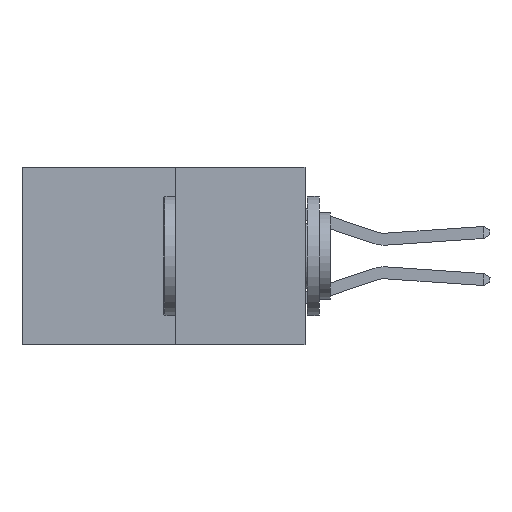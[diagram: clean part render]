
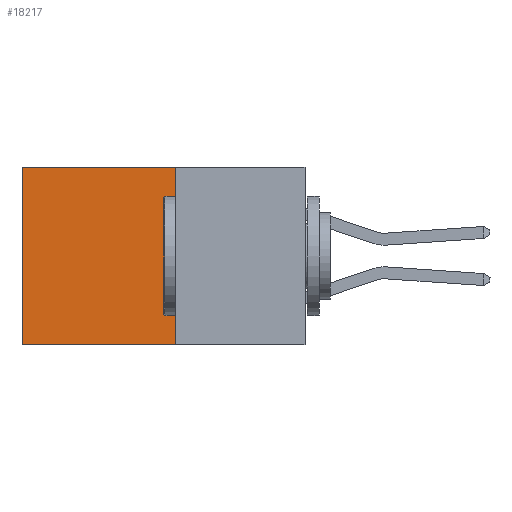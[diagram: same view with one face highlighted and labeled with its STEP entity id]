
A CAD part, left-side view. The second image highlights one B-rep face of the part: STEP entity #18217.
In plain terms, the highlighted planar face has unit normal (-1, 0, 0).
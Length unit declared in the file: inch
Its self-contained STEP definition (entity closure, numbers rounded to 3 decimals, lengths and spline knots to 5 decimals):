
#275 = LINE ( 'NONE', #4402, #13300 ) ;
#378 = VERTEX_POINT ( 'NONE', #5801 ) ;
#997 = EDGE_CURVE ( 'NONE', #378, #18207, #5376, .T. ) ;
#1364 = CARTESIAN_POINT ( 'NONE',  ( 0.277, 0.27, -0.37 ) ) ;
#1734 = VERTEX_POINT ( 'NONE', #11435 ) ;
#1877 = PLANE ( 'NONE',  #4351 ) ;
#1931 = ORIENTED_EDGE ( 'NONE', *, *, #997, .F. ) ;
#3679 = VERTEX_POINT ( 'NONE', #12631 ) ;
#4232 = LINE ( 'NONE', #15502, #8170 ) ;
#4351 = AXIS2_PLACEMENT_3D ( 'NONE', #5242, #17180, #6920 ) ;
#4374 = ORIENTED_EDGE ( 'NONE', *, *, #11932, .F. ) ;
#4402 = CARTESIAN_POINT ( 'NONE',  ( 0.277, 0.27, 0. ) ) ;
#4960 = DIRECTION ( 'NONE',  ( 0., 0., -1. ) ) ;
#5242 = CARTESIAN_POINT ( 'NONE',  ( 0.277, 0.27, -0.37 ) ) ;
#5376 = LINE ( 'NONE', #1364, #18435 ) ;
#5501 = VECTOR ( 'NONE', #4960, 39.37008 ) ;
#5801 = CARTESIAN_POINT ( 'NONE',  ( 0.277, 0.27, 0. ) ) ;
#6067 = DIRECTION ( 'NONE',  ( 0., 1., 0. ) ) ;
#6920 = DIRECTION ( 'NONE',  ( 0., 0., -1. ) ) ;
#6954 = DIRECTION ( 'NONE',  ( 0., 1., 0. ) ) ;
#8170 = VECTOR ( 'NONE', #6954, 39.37008 ) ;
#9009 = ORIENTED_EDGE ( 'NONE', *, *, #12502, .T. ) ;
#9467 = LINE ( 'NONE', #15188, #5501 ) ;
#10006 = EDGE_LOOP ( 'NONE', ( #9009, #4374, #1931, #21044 ) ) ;
#11435 = CARTESIAN_POINT ( 'NONE',  ( 0.277, 0.59, -0.37 ) ) ;
#11932 = EDGE_CURVE ( 'NONE', #18207, #1734, #4232, .T. ) ;
#12502 = EDGE_CURVE ( 'NONE', #3679, #1734, #9467, .T. ) ;
#12631 = CARTESIAN_POINT ( 'NONE',  ( 0.277, 0.59, 0. ) ) ;
#13300 = VECTOR ( 'NONE', #6067, 39.37008 ) ;
#13715 = EDGE_CURVE ( 'NONE', #378, #3679, #275, .T. ) ;
#15188 = CARTESIAN_POINT ( 'NONE',  ( 0.277, 0.59, -0.37 ) ) ;
#15502 = CARTESIAN_POINT ( 'NONE',  ( 0.277, 0.27, -0.37 ) ) ;
#17110 = CARTESIAN_POINT ( 'NONE',  ( 0.277, 0.27, -0.37 ) ) ;
#17180 = DIRECTION ( 'NONE',  ( 1., 0., 0. ) ) ;
#17909 = FACE_OUTER_BOUND ( 'NONE', #10006, .T. ) ;
#18207 = VERTEX_POINT ( 'NONE', #17110 ) ;
#18217 = ADVANCED_FACE ( 'NONE', ( #17909 ), #1877, .F. ) ;
#18435 = VECTOR ( 'NONE', #20905, 39.37008 ) ;
#20905 = DIRECTION ( 'NONE',  ( 0., 0., -1. ) ) ;
#21044 = ORIENTED_EDGE ( 'NONE', *, *, #13715, .T. ) ;
